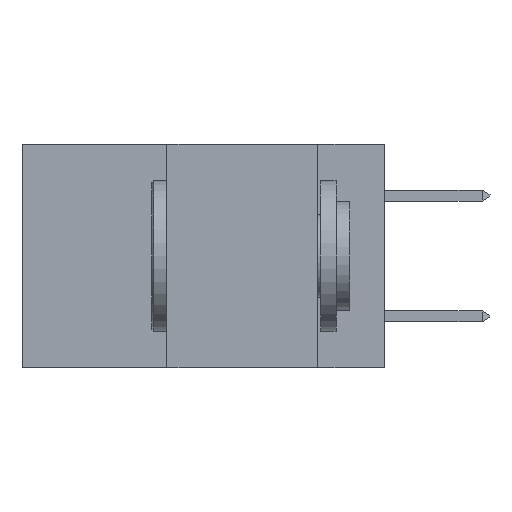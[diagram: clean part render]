
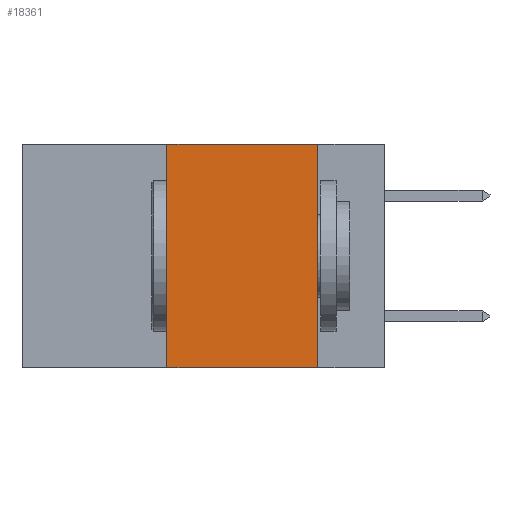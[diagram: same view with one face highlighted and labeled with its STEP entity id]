
A CAD part, left-side view. The second image highlights one B-rep face of the part: STEP entity #18361.
In plain terms, the highlighted planar face has unit normal (-1, 0, 0).
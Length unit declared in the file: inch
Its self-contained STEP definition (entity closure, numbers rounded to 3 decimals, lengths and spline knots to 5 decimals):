
#758 = VECTOR ( 'NONE', #1984, 39.37008 ) ;
#1984 = DIRECTION ( 'NONE',  ( 0., 0., 1. ) ) ;
#2413 = DIRECTION ( 'NONE',  ( 0., 0., -1. ) ) ;
#4461 = CARTESIAN_POINT ( 'NONE',  ( 0., 0.11, 0. ) ) ;
#5853 = CARTESIAN_POINT ( 'NONE',  ( 0., 0.11, 0. ) ) ;
#6026 = VERTEX_POINT ( 'NONE', #8558 ) ;
#6244 = CARTESIAN_POINT ( 'NONE',  ( 0., 0.11, -0.37 ) ) ;
#6794 = EDGE_CURVE ( 'NONE', #16134, #20442, #8167, .T. ) ;
#7827 = EDGE_CURVE ( 'NONE', #20442, #18521, #11339, .T. ) ;
#8167 = LINE ( 'NONE', #13582, #20662 ) ;
#8558 = CARTESIAN_POINT ( 'NONE',  ( 0., 0.36, -0.37 ) ) ;
#9423 = EDGE_CURVE ( 'NONE', #6026, #16134, #13930, .T. ) ;
#9971 = AXIS2_PLACEMENT_3D ( 'NONE', #19434, #12692, #2413 ) ;
#10381 = LINE ( 'NONE', #19570, #18897 ) ;
#11051 = ORIENTED_EDGE ( 'NONE', *, *, #21626, .T. ) ;
#11339 = LINE ( 'NONE', #4461, #15342 ) ;
#11383 = DIRECTION ( 'NONE',  ( 0., 0., -1. ) ) ;
#12269 = CARTESIAN_POINT ( 'NONE',  ( 0., 0.36, 0. ) ) ;
#12454 = ORIENTED_EDGE ( 'NONE', *, *, #6794, .F. ) ;
#12692 = DIRECTION ( 'NONE',  ( 1., 0., 0. ) ) ;
#13582 = CARTESIAN_POINT ( 'NONE',  ( 0., 0.6, 0. ) ) ;
#13930 = LINE ( 'NONE', #12269, #758 ) ;
#14615 = FACE_OUTER_BOUND ( 'NONE', #14931, .T. ) ;
#14931 = EDGE_LOOP ( 'NONE', ( #16446, #12454, #22044, #11051 ) ) ;
#15295 = DIRECTION ( 'NONE',  ( 0., -1., 0. ) ) ;
#15342 = VECTOR ( 'NONE', #11383, 39.37008 ) ;
#16134 = VERTEX_POINT ( 'NONE', #19738 ) ;
#16446 = ORIENTED_EDGE ( 'NONE', *, *, #7827, .F. ) ;
#17860 = DIRECTION ( 'NONE',  ( 0., -1., 0. ) ) ;
#18361 = ADVANCED_FACE ( 'NONE', ( #14615 ), #21160, .F. ) ;
#18521 = VERTEX_POINT ( 'NONE', #6244 ) ;
#18897 = VECTOR ( 'NONE', #17860, 39.37008 ) ;
#19434 = CARTESIAN_POINT ( 'NONE',  ( 0., 0.6, 0. ) ) ;
#19570 = CARTESIAN_POINT ( 'NONE',  ( 0., 0.6, -0.37 ) ) ;
#19738 = CARTESIAN_POINT ( 'NONE',  ( 0., 0.36, 0. ) ) ;
#20442 = VERTEX_POINT ( 'NONE', #5853 ) ;
#20662 = VECTOR ( 'NONE', #15295, 39.37008 ) ;
#21160 = PLANE ( 'NONE',  #9971 ) ;
#21626 = EDGE_CURVE ( 'NONE', #6026, #18521, #10381, .T. ) ;
#22044 = ORIENTED_EDGE ( 'NONE', *, *, #9423, .F. ) ;
